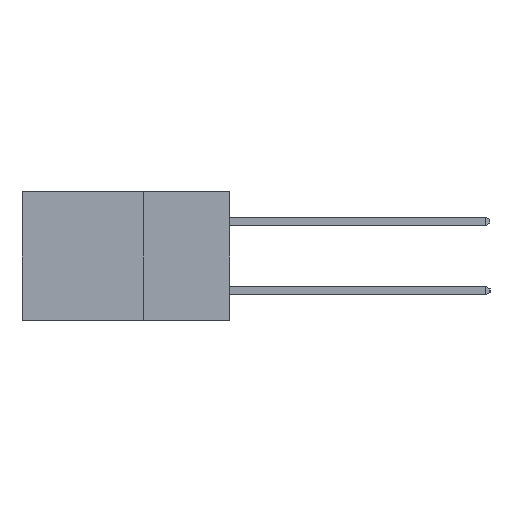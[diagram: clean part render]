
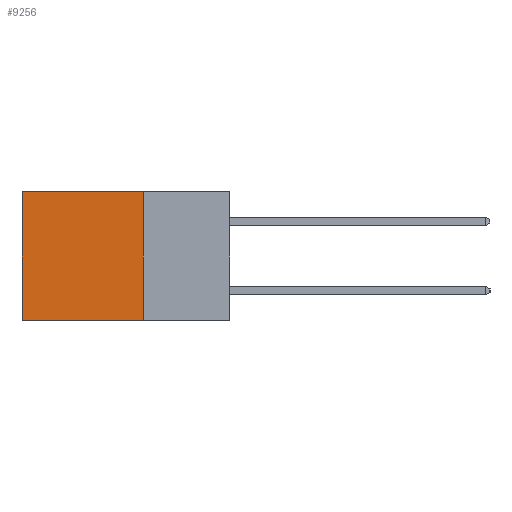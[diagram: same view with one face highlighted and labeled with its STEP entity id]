
A CAD part, left-side view. The second image highlights one B-rep face of the part: STEP entity #9256.
In plain terms, the highlighted planar face has unit normal (-1, 0, 0).
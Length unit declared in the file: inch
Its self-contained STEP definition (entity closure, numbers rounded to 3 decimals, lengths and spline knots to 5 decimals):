
#60 = PLANE ( 'NONE',  #3337 ) ;
#276 = CARTESIAN_POINT ( 'NONE',  ( 0.2615, 0.25, -0.37 ) ) ;
#327 = VERTEX_POINT ( 'NONE', #5820 ) ;
#702 = FACE_OUTER_BOUND ( 'NONE', #8621, .T. ) ;
#989 = VECTOR ( 'NONE', #13025, 39.37008 ) ;
#993 = VECTOR ( 'NONE', #12795, 39.37008 ) ;
#1619 = ORIENTED_EDGE ( 'NONE', *, *, #6183, .T. ) ;
#1773 = CARTESIAN_POINT ( 'NONE',  ( 0.2615, 0.25, 0. ) ) ;
#3110 = LINE ( 'NONE', #14491, #5683 ) ;
#3337 = AXIS2_PLACEMENT_3D ( 'NONE', #276, #14640, #14625 ) ;
#3498 = ORIENTED_EDGE ( 'NONE', *, *, #9267, .F. ) ;
#3818 = VERTEX_POINT ( 'NONE', #7551 ) ;
#4052 = LINE ( 'NONE', #12906, #993 ) ;
#4520 = CARTESIAN_POINT ( 'NONE',  ( 0.2615, 0.25, 0. ) ) ;
#4547 = DIRECTION ( 'NONE',  ( 0., 1., 0. ) ) ;
#5496 = VECTOR ( 'NONE', #4547, 39.37008 ) ;
#5599 = VERTEX_POINT ( 'NONE', #11852 ) ;
#5683 = VECTOR ( 'NONE', #14474, 39.37008 ) ;
#5820 = CARTESIAN_POINT ( 'NONE',  ( 0.2615, 0.6, -0.37 ) ) ;
#6183 = EDGE_CURVE ( 'NONE', #3818, #327, #13233, .T. ) ;
#7551 = CARTESIAN_POINT ( 'NONE',  ( 0.2615, 0.6, 0. ) ) ;
#7681 = ORIENTED_EDGE ( 'NONE', *, *, #10059, .T. ) ;
#8621 = EDGE_LOOP ( 'NONE', ( #1619, #3498, #10512, #7681 ) ) ;
#9208 = VERTEX_POINT ( 'NONE', #1773 ) ;
#9256 = ADVANCED_FACE ( 'NONE', ( #702 ), #60, .F. ) ;
#9267 = EDGE_CURVE ( 'NONE', #5599, #327, #3110, .T. ) ;
#10059 = EDGE_CURVE ( 'NONE', #9208, #3818, #14260, .T. ) ;
#10512 = ORIENTED_EDGE ( 'NONE', *, *, #13259, .F. ) ;
#11852 = CARTESIAN_POINT ( 'NONE',  ( 0.2615, 0.25, -0.37 ) ) ;
#12795 = DIRECTION ( 'NONE',  ( 0., 0., -1. ) ) ;
#12906 = CARTESIAN_POINT ( 'NONE',  ( 0.2615, 0.25, -0.37 ) ) ;
#13025 = DIRECTION ( 'NONE',  ( 0., 0., -1. ) ) ;
#13149 = CARTESIAN_POINT ( 'NONE',  ( 0.2615, 0.6, -0.37 ) ) ;
#13233 = LINE ( 'NONE', #13149, #989 ) ;
#13259 = EDGE_CURVE ( 'NONE', #9208, #5599, #4052, .T. ) ;
#14260 = LINE ( 'NONE', #4520, #5496 ) ;
#14474 = DIRECTION ( 'NONE',  ( 0., 1., 0. ) ) ;
#14491 = CARTESIAN_POINT ( 'NONE',  ( 0.2615, 0.25, -0.37 ) ) ;
#14625 = DIRECTION ( 'NONE',  ( 0., 0., -1. ) ) ;
#14640 = DIRECTION ( 'NONE',  ( 1., 0., 0. ) ) ;
